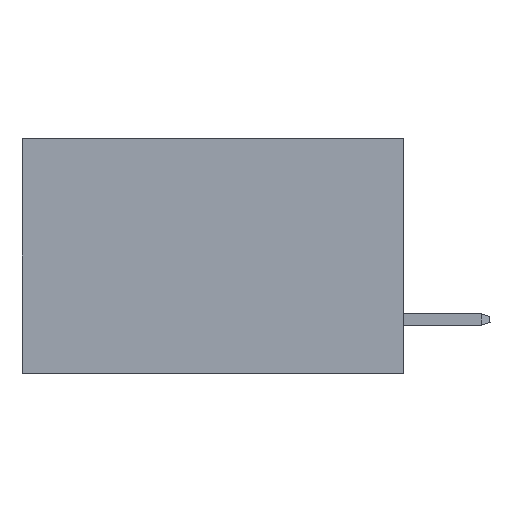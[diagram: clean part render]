
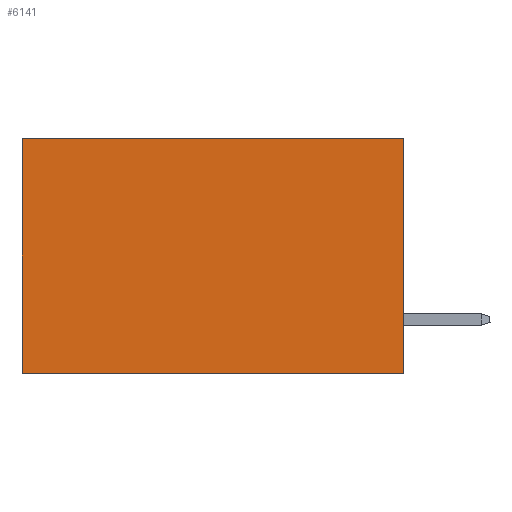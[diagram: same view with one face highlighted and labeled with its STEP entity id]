
A CAD part, left-side view. The second image highlights one B-rep face of the part: STEP entity #6141.
In plain terms, the highlighted planar face has unit normal (-1, 0, 0).
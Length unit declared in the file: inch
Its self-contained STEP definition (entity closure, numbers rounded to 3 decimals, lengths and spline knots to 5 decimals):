
#224 = ORIENTED_EDGE ( 'NONE', *, *, #17308, .F. ) ;
#576 = VERTEX_POINT ( 'NONE', #4665 ) ;
#736 = CARTESIAN_POINT ( 'NONE',  ( 0.2875, 0., 0. ) ) ;
#1268 = ORIENTED_EDGE ( 'NONE', *, *, #18189, .T. ) ;
#3867 = DIRECTION ( 'NONE',  ( 0., 1., 0. ) ) ;
#4558 = FACE_OUTER_BOUND ( 'NONE', #11459, .T. ) ;
#4665 = CARTESIAN_POINT ( 'NONE',  ( 0.2875, 0., -0.37 ) ) ;
#4780 = CARTESIAN_POINT ( 'NONE',  ( 0.2875, 0., 0. ) ) ;
#5017 = LINE ( 'NONE', #11194, #17500 ) ;
#5206 = LINE ( 'NONE', #17091, #13788 ) ;
#5221 = LINE ( 'NONE', #8035, #16039 ) ;
#5259 = VECTOR ( 'NONE', #14011, 39.37008 ) ;
#5546 = VERTEX_POINT ( 'NONE', #9297 ) ;
#6141 = ADVANCED_FACE ( 'NONE', ( #4558 ), #10479, .F. ) ;
#7299 = ORIENTED_EDGE ( 'NONE', *, *, #10022, .T. ) ;
#7602 = ORIENTED_EDGE ( 'NONE', *, *, #11067, .F. ) ;
#8035 = CARTESIAN_POINT ( 'NONE',  ( 0.2875, 0., 0. ) ) ;
#9207 = VERTEX_POINT ( 'NONE', #4780 ) ;
#9297 = CARTESIAN_POINT ( 'NONE',  ( 0.2875, 0.6, -0.37 ) ) ;
#9512 = CARTESIAN_POINT ( 'NONE',  ( 0.2875, 0.6, 0. ) ) ;
#10022 = EDGE_CURVE ( 'NONE', #12049, #5546, #5017, .T. ) ;
#10479 = PLANE ( 'NONE',  #13701 ) ;
#10920 = DIRECTION ( 'NONE',  ( 0., 0., -1. ) ) ;
#11030 = LINE ( 'NONE', #18744, #5259 ) ;
#11067 = EDGE_CURVE ( 'NONE', #576, #5546, #5206, .T. ) ;
#11194 = CARTESIAN_POINT ( 'NONE',  ( 0.2875, 0.6, 0. ) ) ;
#11459 = EDGE_LOOP ( 'NONE', ( #7299, #7602, #224, #1268 ) ) ;
#12049 = VERTEX_POINT ( 'NONE', #9512 ) ;
#12460 = DIRECTION ( 'NONE',  ( 0., 0., -1. ) ) ;
#13701 = AXIS2_PLACEMENT_3D ( 'NONE', #736, #18371, #16746 ) ;
#13788 = VECTOR ( 'NONE', #3867, 39.37008 ) ;
#14011 = DIRECTION ( 'NONE',  ( 0., 1., 0. ) ) ;
#16039 = VECTOR ( 'NONE', #12460, 39.37008 ) ;
#16746 = DIRECTION ( 'NONE',  ( 0., 0., -1. ) ) ;
#17091 = CARTESIAN_POINT ( 'NONE',  ( 0.2875, 0., -0.37 ) ) ;
#17308 = EDGE_CURVE ( 'NONE', #9207, #576, #5221, .T. ) ;
#17500 = VECTOR ( 'NONE', #10920, 39.37008 ) ;
#18189 = EDGE_CURVE ( 'NONE', #9207, #12049, #11030, .T. ) ;
#18371 = DIRECTION ( 'NONE',  ( 1., 0., 0. ) ) ;
#18744 = CARTESIAN_POINT ( 'NONE',  ( 0.2875, 0., 0. ) ) ;
